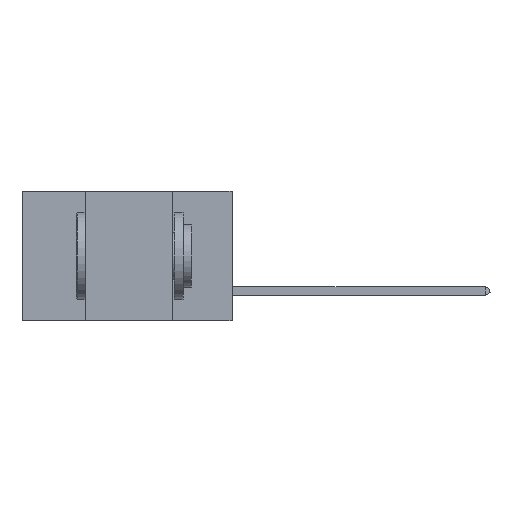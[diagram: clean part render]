
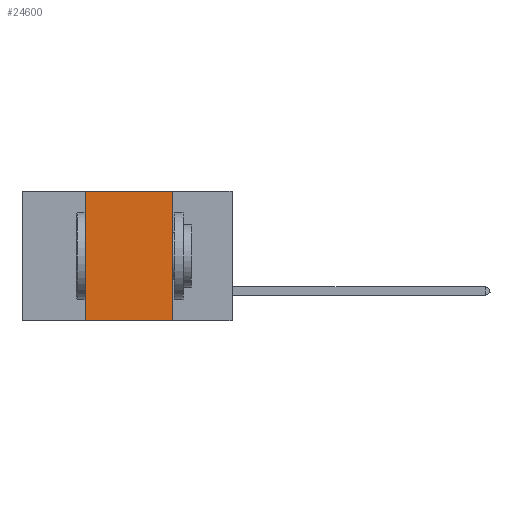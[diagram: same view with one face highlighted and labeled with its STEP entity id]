
A CAD part, left-side view. The second image highlights one B-rep face of the part: STEP entity #24600.
In plain terms, the highlighted planar face has unit normal (-1, 0, 0).
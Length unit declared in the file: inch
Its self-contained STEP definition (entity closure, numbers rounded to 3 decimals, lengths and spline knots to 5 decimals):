
#222 = DIRECTION ( 'NONE',  ( 0., 0., 1. ) ) ;
#4241 = ORIENTED_EDGE ( 'NONE', *, *, #28291, .F. ) ;
#6248 = CARTESIAN_POINT ( 'NONE',  ( 0., 0.17, 0. ) ) ;
#6307 = PLANE ( 'NONE',  #32049 ) ;
#6552 = ORIENTED_EDGE ( 'NONE', *, *, #8230, .F. ) ;
#6703 = LINE ( 'NONE', #18687, #27984 ) ;
#8230 = EDGE_CURVE ( 'NONE', #29319, #44532, #39340, .T. ) ;
#10252 = VERTEX_POINT ( 'NONE', #12209 ) ;
#10582 = CARTESIAN_POINT ( 'NONE',  ( 0., 0.42, 0. ) ) ;
#11338 = VERTEX_POINT ( 'NONE', #21618 ) ;
#11368 = CARTESIAN_POINT ( 'NONE',  ( 0., 0.17, -0.37 ) ) ;
#11880 = ORIENTED_EDGE ( 'NONE', *, *, #20999, .F. ) ;
#12209 = CARTESIAN_POINT ( 'NONE',  ( 0., 0.42, -0.37 ) ) ;
#13327 = DIRECTION ( 'NONE',  ( 1., 0., 0. ) ) ;
#16389 = FACE_OUTER_BOUND ( 'NONE', #38705, .T. ) ;
#18507 = VECTOR ( 'NONE', #22008, 39.37008 ) ;
#18687 = CARTESIAN_POINT ( 'NONE',  ( 0., 0.6, -0.37 ) ) ;
#19819 = DIRECTION ( 'NONE',  ( 0., 0., -1. ) ) ;
#19948 = VECTOR ( 'NONE', #222, 39.37008 ) ;
#20999 = EDGE_CURVE ( 'NONE', #10252, #11338, #38504, .T. ) ;
#21618 = CARTESIAN_POINT ( 'NONE',  ( 0., 0.42, 0. ) ) ;
#22008 = DIRECTION ( 'NONE',  ( 0., -1., 0. ) ) ;
#22171 = CARTESIAN_POINT ( 'NONE',  ( 0., 0.6, 0. ) ) ;
#22966 = VECTOR ( 'NONE', #40718, 39.37008 ) ;
#24600 = ADVANCED_FACE ( 'NONE', ( #16389 ), #6307, .F. ) ;
#27984 = VECTOR ( 'NONE', #29278, 39.37008 ) ;
#28291 = EDGE_CURVE ( 'NONE', #11338, #29319, #28964, .T. ) ;
#28964 = LINE ( 'NONE', #22171, #18507 ) ;
#29278 = DIRECTION ( 'NONE',  ( 0., -1., 0. ) ) ;
#29319 = VERTEX_POINT ( 'NONE', #39338 ) ;
#32049 = AXIS2_PLACEMENT_3D ( 'NONE', #37249, #13327, #19819 ) ;
#35985 = EDGE_CURVE ( 'NONE', #10252, #44532, #6703, .T. ) ;
#37249 = CARTESIAN_POINT ( 'NONE',  ( 0., 0.6, 0. ) ) ;
#38504 = LINE ( 'NONE', #10582, #19948 ) ;
#38705 = EDGE_LOOP ( 'NONE', ( #6552, #4241, #11880, #39583 ) ) ;
#39338 = CARTESIAN_POINT ( 'NONE',  ( 0., 0.17, 0. ) ) ;
#39340 = LINE ( 'NONE', #6248, #22966 ) ;
#39583 = ORIENTED_EDGE ( 'NONE', *, *, #35985, .T. ) ;
#40718 = DIRECTION ( 'NONE',  ( 0., 0., -1. ) ) ;
#44532 = VERTEX_POINT ( 'NONE', #11368 ) ;
